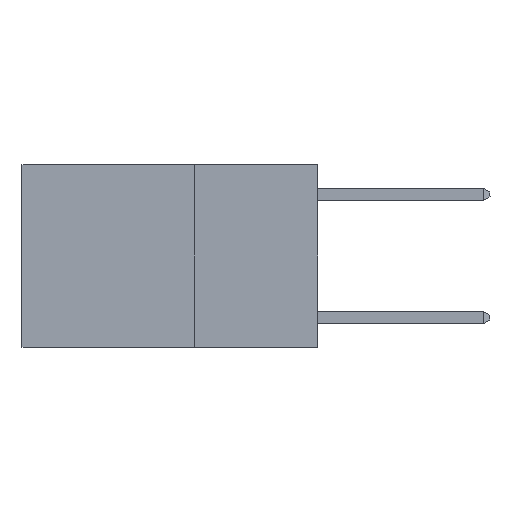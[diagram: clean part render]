
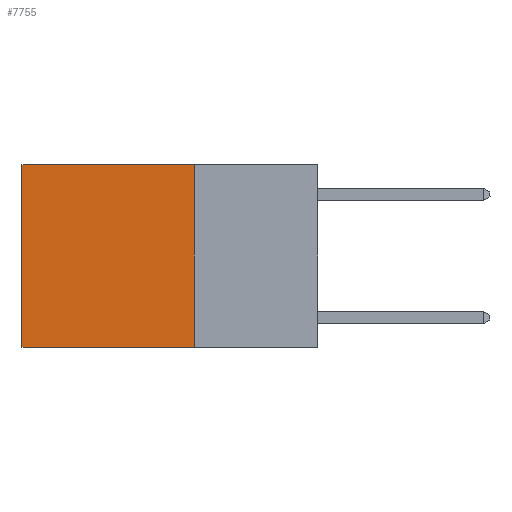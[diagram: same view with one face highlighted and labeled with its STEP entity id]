
A CAD part, left-side view. The second image highlights one B-rep face of the part: STEP entity #7755.
In plain terms, the highlighted planar face has unit normal (-1, 0, 0).
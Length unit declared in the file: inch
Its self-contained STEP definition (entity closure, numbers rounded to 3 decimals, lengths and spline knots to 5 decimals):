
#247 = ORIENTED_EDGE ( 'NONE', *, *, #5976, .F. ) ;
#355 = AXIS2_PLACEMENT_3D ( 'NONE', #4041, #9212, #9315 ) ;
#619 = ORIENTED_EDGE ( 'NONE', *, *, #8157, .T. ) ;
#657 = VERTEX_POINT ( 'NONE', #5788 ) ;
#669 = EDGE_CURVE ( 'NONE', #657, #2987, #2930, .T. ) ;
#876 = CARTESIAN_POINT ( 'NONE',  ( 0.2625, 0.25, 0. ) ) ;
#884 = LINE ( 'NONE', #3085, #8346 ) ;
#888 = ORIENTED_EDGE ( 'NONE', *, *, #3102, .F. ) ;
#1241 = CARTESIAN_POINT ( 'NONE',  ( 0.2625, 0.25, -0.37 ) ) ;
#1414 = VECTOR ( 'NONE', #9324, 39.37008 ) ;
#1593 = LINE ( 'NONE', #876, #5449 ) ;
#2622 = ORIENTED_EDGE ( 'NONE', *, *, #669, .T. ) ;
#2930 = LINE ( 'NONE', #5977, #7288 ) ;
#2942 = DIRECTION ( 'NONE',  ( 0., 1., 0. ) ) ;
#2987 = VERTEX_POINT ( 'NONE', #8225 ) ;
#3085 = CARTESIAN_POINT ( 'NONE',  ( 0.2625, 0.25, -0.37 ) ) ;
#3102 = EDGE_CURVE ( 'NONE', #5155, #2987, #884, .T. ) ;
#3315 = FACE_OUTER_BOUND ( 'NONE', #6746, .T. ) ;
#3808 = DIRECTION ( 'NONE',  ( 0., 1., 0. ) ) ;
#4041 = CARTESIAN_POINT ( 'NONE',  ( 0.2625, 0.25, 0. ) ) ;
#4834 = LINE ( 'NONE', #4986, #1414 ) ;
#4973 = PLANE ( 'NONE',  #355 ) ;
#4986 = CARTESIAN_POINT ( 'NONE',  ( 0.2625, 0.25, 0. ) ) ;
#5155 = VERTEX_POINT ( 'NONE', #1241 ) ;
#5449 = VECTOR ( 'NONE', #3808, 39.37008 ) ;
#5788 = CARTESIAN_POINT ( 'NONE',  ( 0.2625, 0.6, 0. ) ) ;
#5976 = EDGE_CURVE ( 'NONE', #7793, #5155, #4834, .T. ) ;
#5977 = CARTESIAN_POINT ( 'NONE',  ( 0.2625, 0.6, 0. ) ) ;
#6313 = CARTESIAN_POINT ( 'NONE',  ( 0.2625, 0.25, 0. ) ) ;
#6746 = EDGE_LOOP ( 'NONE', ( #2622, #888, #247, #619 ) ) ;
#7288 = VECTOR ( 'NONE', #8116, 39.37008 ) ;
#7755 = ADVANCED_FACE ( 'NONE', ( #3315 ), #4973, .F. ) ;
#7793 = VERTEX_POINT ( 'NONE', #6313 ) ;
#8116 = DIRECTION ( 'NONE',  ( 0., 0., -1. ) ) ;
#8157 = EDGE_CURVE ( 'NONE', #7793, #657, #1593, .T. ) ;
#8225 = CARTESIAN_POINT ( 'NONE',  ( 0.2625, 0.6, -0.37 ) ) ;
#8346 = VECTOR ( 'NONE', #2942, 39.37008 ) ;
#9212 = DIRECTION ( 'NONE',  ( 1., 0., 0. ) ) ;
#9315 = DIRECTION ( 'NONE',  ( 0., 0., -1. ) ) ;
#9324 = DIRECTION ( 'NONE',  ( 0., 0., -1. ) ) ;
